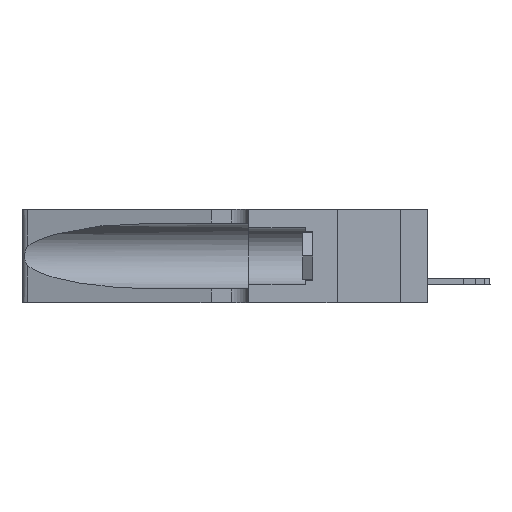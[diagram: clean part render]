
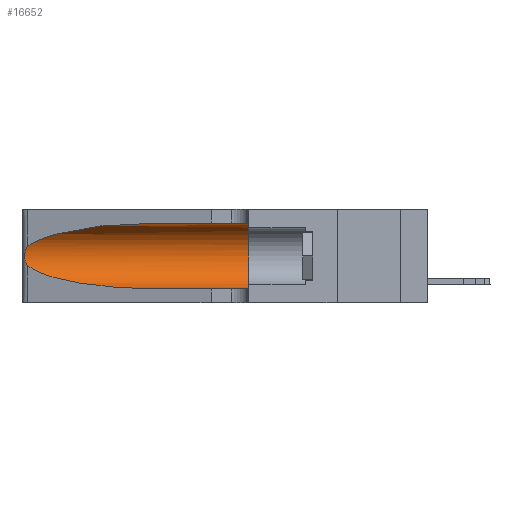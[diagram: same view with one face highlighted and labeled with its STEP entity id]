
A CAD part, left-side view. The second image highlights one B-rep face of the part: STEP entity #16652.
In plain terms, the highlighted cylindrical face has radius 3.308 mm (diameter 6.617 mm), a partial arc.
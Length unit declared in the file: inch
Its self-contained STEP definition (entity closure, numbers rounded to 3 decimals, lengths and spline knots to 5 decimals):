
#270 = EDGE_CURVE ( 'NONE', #17778, #26182, #28460, .T. ) ;
#1524 = CARTESIAN_POINT ( 'NONE',  ( 0.2373, 1.15595, 0.28018 ) ) ;
#3914 = VECTOR ( 'NONE', #35181, 39.37008 ) ;
#4242 = EDGE_CURVE ( 'NONE', #17778, #30757, #25288, .T. ) ;
#4289 = DIRECTION ( 'NONE',  ( 0., -1., 0. ) ) ;
#4324 = CARTESIAN_POINT ( 'NONE',  ( 0.25639, 1.23184, 0.21858 ) ) ;
#4809 = CARTESIAN_POINT ( 'NONE',  ( 0.25555, 1.22993, 0.14849 ) ) ;
#7242 = CARTESIAN_POINT ( 'NONE',  ( 0.25787, 1.23484, 0.2124 ) ) ;
#7335 = DIRECTION ( 'NONE',  ( 0., 0., -1. ) ) ;
#7365 = CYLINDRICAL_SURFACE ( 'NONE', #25369, 0.13025 ) ;
#7575 = EDGE_LOOP ( 'NONE', ( #37187, #31895, #34958, #30044, #12288, #23306 ) ) ;
#10422 = CARTESIAN_POINT ( 'NONE',  ( 0.25854, 1.2359, 0.20912 ) ) ;
#10487 = CARTESIAN_POINT ( 'NONE',  ( 0.1305, 0.72297, 0.05475 ) ) ;
#10883 = DIRECTION ( 'NONE',  ( 0., 1., 0. ) ) ;
#12288 = ORIENTED_EDGE ( 'NONE', *, *, #23748, .F. ) ;
#12455 = CARTESIAN_POINT ( 'NONE',  ( 0.1305, 0.72297, 0.05475 ) ) ;
#12937 = CARTESIAN_POINT ( 'NONE',  ( 0.1305, 0.72297, 0.31525 ) ) ;
#13090 = CARTESIAN_POINT ( 'NONE',  ( 0.25487, 1.22718, 0.22369 ) ) ;
#14632 = FACE_OUTER_BOUND ( 'NONE', #7575, .T. ) ;
#15090 = CARTESIAN_POINT ( 'NONE',  ( 0.1305, 1.61858, 0.05475 ) ) ;
#15321 = AXIS2_PLACEMENT_3D ( 'NONE', #16631, #10883, #19708 ) ;
#15428 = VERTEX_POINT ( 'NONE', #10487 ) ;
#16455 = CARTESIAN_POINT ( 'NONE',  ( 0.1305, 0.35, 0.05475 ) ) ;
#16631 = CARTESIAN_POINT ( 'NONE',  ( 0.1305, 0.35, 0.185 ) ) ;
#16652 = ADVANCED_FACE ( 'NONE', ( #14632 ), #7365, .F. ) ;
#17508 = VERTEX_POINT ( 'NONE', #23970 ) ;
#17778 = VERTEX_POINT ( 'NONE', #24506 ) ;
#18674 = CARTESIAN_POINT ( 'NONE',  ( 0.1305, 1.61858, 0.185 ) ) ;
#18978 = CARTESIAN_POINT ( 'NONE',  ( 0.26075, 1.23896, 0.178 ) ) ;
#19708 = DIRECTION ( 'NONE',  ( 0., 0., 1. ) ) ;
#19852 = CARTESIAN_POINT ( 'NONE',  ( 0.25789, 1.23486, 0.15765 ) ) ;
#21738 = CARTESIAN_POINT ( 'NONE',  ( 0.25555, 1.22994, 0.2215 ) ) ;
#21848 = CARTESIAN_POINT ( 'NONE',  ( 0.25487, 1.22718, 0.22369 ) ) ;
#21859 = CARTESIAN_POINT ( 'NONE',  ( 0.25856, 1.23593, 0.16098 ) ) ;
#23087 = CARTESIAN_POINT ( 'NONE',  ( 0.1305, 1.61858, 0.31525 ) ) ;
#23306 = ORIENTED_EDGE ( 'NONE', *, *, #270, .F. ) ;
#23748 = EDGE_CURVE ( 'NONE', #26182, #33665, #27369, .T. ) ;
#23870 = CARTESIAN_POINT ( 'NONE',  ( 0.25487, 1.22718, 0.14631 ) ) ;
#23970 = CARTESIAN_POINT ( 'NONE',  ( 0.25487, 1.22718, 0.14631 ) ) ;
#24094 =( BOUNDED_CURVE ( )  B_SPLINE_CURVE ( 3, ( #23870, #26779, #29650, #12455 ),
 .UNSPECIFIED., .F., .T. ) 
 B_SPLINE_CURVE_WITH_KNOTS ( ( 4, 4 ),
 ( 3.44316, 4.71239 ),
 .UNSPECIFIED. ) 
 CURVE ( )  GEOMETRIC_REPRESENTATION_ITEM ( )  RATIONAL_B_SPLINE_CURVE ( ( 1., 0.87, 0.87, 1. ) ) 
 REPRESENTATION_ITEM ( '' )  );
#24506 = CARTESIAN_POINT ( 'NONE',  ( 0.1305, 0.72297, 0.31525 ) ) ;
#25288 =( BOUNDED_CURVE ( )  B_SPLINE_CURVE ( 3, ( #12937, #27504, #1524, #21848 ),
 .UNSPECIFIED., .F., .T. ) 
 B_SPLINE_CURVE_WITH_KNOTS ( ( 4, 4 ),
 ( 1.5708, 2.84003 ),
 .UNSPECIFIED. ) 
 CURVE ( )  GEOMETRIC_REPRESENTATION_ITEM ( )  RATIONAL_B_SPLINE_CURVE ( ( 1., 0.87, 0.87, 1. ) ) 
 REPRESENTATION_ITEM ( '' )  );
#25369 = AXIS2_PLACEMENT_3D ( 'NONE', #18674, #4289, #7335 ) ;
#25713 = B_SPLINE_CURVE_WITH_KNOTS ( 'NONE', 3,
 ( #27261, #21738, #4324, #7242, #10422, #27528, #33343, #18978, #30666, #21859, #19852, #31305, #4809, #33981 ),
 .UNSPECIFIED., .F., .F.,
 ( 4, 2, 2, 2, 2, 2, 4 ),
 ( 0., 0.00027, 0.00053, 0.00107, 0.0016, 0.00187, 0.00214 ),
 .UNSPECIFIED. ) ;
#26169 = EDGE_CURVE ( 'NONE', #17508, #15428, #24094, .T. ) ;
#26182 = VERTEX_POINT ( 'NONE', #34987 ) ;
#26779 = CARTESIAN_POINT ( 'NONE',  ( 0.2373, 1.15595, 0.08982 ) ) ;
#27261 = CARTESIAN_POINT ( 'NONE',  ( 0.25487, 1.22718, 0.22369 ) ) ;
#27369 = CIRCLE ( 'NONE', #15321, 0.13025 ) ;
#27504 = CARTESIAN_POINT ( 'NONE',  ( 0.18966, 0.96281, 0.31525 ) ) ;
#27528 = CARTESIAN_POINT ( 'NONE',  ( 0.26018, 1.23835, 0.19895 ) ) ;
#28460 = LINE ( 'NONE', #23087, #28880 ) ;
#28856 = EDGE_CURVE ( 'NONE', #30757, #17508, #25713, .T. ) ;
#28880 = VECTOR ( 'NONE', #34804, 39.37008 ) ;
#29650 = CARTESIAN_POINT ( 'NONE',  ( 0.18966, 0.96281, 0.05475 ) ) ;
#30044 = ORIENTED_EDGE ( 'NONE', *, *, #36542, .T. ) ;
#30666 = CARTESIAN_POINT ( 'NONE',  ( 0.26017, 1.23833, 0.17102 ) ) ;
#30675 = LINE ( 'NONE', #15090, #3914 ) ;
#30757 = VERTEX_POINT ( 'NONE', #13090 ) ;
#31305 = CARTESIAN_POINT ( 'NONE',  ( 0.25639, 1.23186, 0.15144 ) ) ;
#31895 = ORIENTED_EDGE ( 'NONE', *, *, #28856, .T. ) ;
#33343 = CARTESIAN_POINT ( 'NONE',  ( 0.26075, 1.23896, 0.19203 ) ) ;
#33665 = VERTEX_POINT ( 'NONE', #16455 ) ;
#33981 = CARTESIAN_POINT ( 'NONE',  ( 0.25487, 1.22718, 0.14631 ) ) ;
#34804 = DIRECTION ( 'NONE',  ( 0., -1., 0. ) ) ;
#34958 = ORIENTED_EDGE ( 'NONE', *, *, #26169, .T. ) ;
#34987 = CARTESIAN_POINT ( 'NONE',  ( 0.1305, 0.35, 0.31525 ) ) ;
#35181 = DIRECTION ( 'NONE',  ( 0., -1., 0. ) ) ;
#36542 = EDGE_CURVE ( 'NONE', #15428, #33665, #30675, .T. ) ;
#37187 = ORIENTED_EDGE ( 'NONE', *, *, #4242, .T. ) ;
